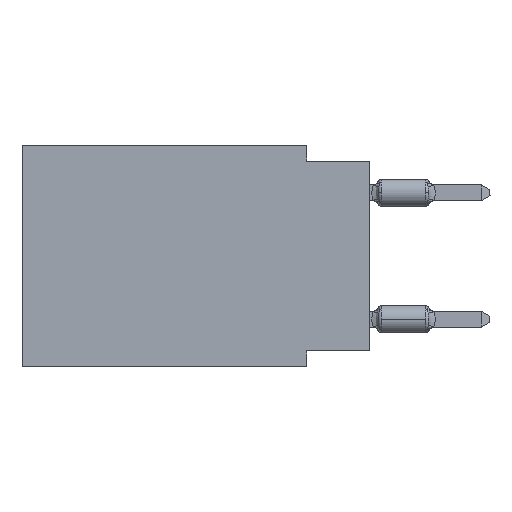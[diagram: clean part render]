
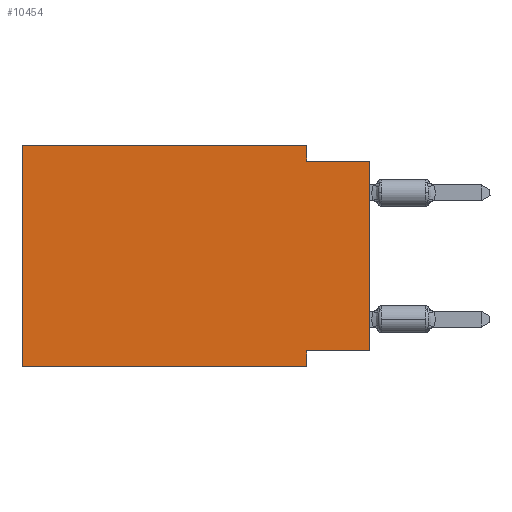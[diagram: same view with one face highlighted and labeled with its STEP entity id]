
A CAD part, left-side view. The second image highlights one B-rep face of the part: STEP entity #10454.
In plain terms, the highlighted planar face has unit normal (-1, 0, 0).
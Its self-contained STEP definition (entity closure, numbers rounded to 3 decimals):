
#143 = VERTEX_POINT ( 'NONE', #18710 ) ;
#406 = LINE ( 'NONE', #12605, #15432 ) ;
#486 = CARTESIAN_POINT ( 'NONE',  ( 0., 0., -0.635 ) ) ;
#492 = VERTEX_POINT ( 'NONE', #29308 ) ;
#1200 = VECTOR ( 'NONE', #30623, 1000. ) ;
#2430 = EDGE_CURVE ( 'NONE', #11170, #37074, #37543, .T. ) ;
#3896 = CARTESIAN_POINT ( 'NONE',  ( 0., 13.97, -8.89 ) ) ;
#4516 = CARTESIAN_POINT ( 'NONE',  ( 0., 0., -8.255 ) ) ;
#5131 = EDGE_CURVE ( 'NONE', #34781, #492, #18862, .T. ) ;
#5402 = AXIS2_PLACEMENT_3D ( 'NONE', #24489, #18121, #9792 ) ;
#5434 = EDGE_LOOP ( 'NONE', ( #22958, #25576, #11327, #9521, #13506, #20418, #31137, #16012 ) ) ;
#5705 = EDGE_CURVE ( 'NONE', #37074, #34781, #22876, .T. ) ;
#5917 = CARTESIAN_POINT ( 'NONE',  ( 0., 13.97, -8.89 ) ) ;
#6017 = CARTESIAN_POINT ( 'NONE',  ( 0., 2.54, -8.89 ) ) ;
#7049 = VERTEX_POINT ( 'NONE', #6017 ) ;
#7102 = EDGE_CURVE ( 'NONE', #143, #7049, #406, .T. ) ;
#8072 = LINE ( 'NONE', #31055, #16519 ) ;
#9521 = ORIENTED_EDGE ( 'NONE', *, *, #2430, .F. ) ;
#9792 = DIRECTION ( 'NONE',  ( 0., 0., -1. ) ) ;
#10207 = CARTESIAN_POINT ( 'NONE',  ( 0., 0., 0. ) ) ;
#10303 = VERTEX_POINT ( 'NONE', #5917 ) ;
#10408 = VECTOR ( 'NONE', #34640, 1000. ) ;
#10454 = ADVANCED_FACE ( 'NONE', ( #32782 ), #12705, .F. ) ;
#10768 = VECTOR ( 'NONE', #13719, 1000. ) ;
#11170 = VERTEX_POINT ( 'NONE', #36300 ) ;
#11327 = ORIENTED_EDGE ( 'NONE', *, *, #5705, .F. ) ;
#12092 = VECTOR ( 'NONE', #13830, 1000. ) ;
#12288 = EDGE_CURVE ( 'NONE', #10303, #7049, #24603, .T. ) ;
#12605 = CARTESIAN_POINT ( 'NONE',  ( 0., 2.54, -8.89 ) ) ;
#12705 = PLANE ( 'NONE',  #5402 ) ;
#13506 = ORIENTED_EDGE ( 'NONE', *, *, #32678, .F. ) ;
#13719 = DIRECTION ( 'NONE',  ( 0., 0., 1. ) ) ;
#13830 = DIRECTION ( 'NONE',  ( 0., 1., 0. ) ) ;
#15386 = CARTESIAN_POINT ( 'NONE',  ( 0., 2.54, 0. ) ) ;
#15432 = VECTOR ( 'NONE', #29792, 1000. ) ;
#16012 = ORIENTED_EDGE ( 'NONE', *, *, #35988, .F. ) ;
#16519 = VECTOR ( 'NONE', #19879, 1000. ) ;
#17059 = CARTESIAN_POINT ( 'NONE',  ( 0., 2.54, 0. ) ) ;
#17237 = VECTOR ( 'NONE', #27504, 1000. ) ;
#18121 = DIRECTION ( 'NONE',  ( 1., 0., 0. ) ) ;
#18710 = CARTESIAN_POINT ( 'NONE',  ( 0., 2.54, -8.255 ) ) ;
#18862 = LINE ( 'NONE', #486, #1200 ) ;
#18929 = VECTOR ( 'NONE', #29420, 1000. ) ;
#19518 = CARTESIAN_POINT ( 'NONE',  ( 0., 0., -8.255 ) ) ;
#19879 = DIRECTION ( 'NONE',  ( 0., 0., 1. ) ) ;
#19963 = VERTEX_POINT ( 'NONE', #19518 ) ;
#20418 = ORIENTED_EDGE ( 'NONE', *, *, #12288, .T. ) ;
#22876 = LINE ( 'NONE', #17059, #10408 ) ;
#22958 = ORIENTED_EDGE ( 'NONE', *, *, #30238, .T. ) ;
#24489 = CARTESIAN_POINT ( 'NONE',  ( 0., 13.97, 0. ) ) ;
#24603 = LINE ( 'NONE', #3896, #17237 ) ;
#25576 = ORIENTED_EDGE ( 'NONE', *, *, #5131, .F. ) ;
#27504 = DIRECTION ( 'NONE',  ( 0., -1., 0. ) ) ;
#29308 = CARTESIAN_POINT ( 'NONE',  ( 0., 0., -0.635 ) ) ;
#29420 = DIRECTION ( 'NONE',  ( 0., -1., 0. ) ) ;
#29792 = DIRECTION ( 'NONE',  ( 0., 0., -1. ) ) ;
#30238 = EDGE_CURVE ( 'NONE', #19963, #492, #31058, .T. ) ;
#30623 = DIRECTION ( 'NONE',  ( 0., -1., 0. ) ) ;
#30785 = CARTESIAN_POINT ( 'NONE',  ( 0., 2.54, -0.635 ) ) ;
#31055 = CARTESIAN_POINT ( 'NONE',  ( 0., 13.97, 0. ) ) ;
#31058 = LINE ( 'NONE', #10207, #10768 ) ;
#31137 = ORIENTED_EDGE ( 'NONE', *, *, #7102, .F. ) ;
#32678 = EDGE_CURVE ( 'NONE', #10303, #11170, #8072, .T. ) ;
#32782 = FACE_OUTER_BOUND ( 'NONE', #5434, .T. ) ;
#34640 = DIRECTION ( 'NONE',  ( 0., 0., -1. ) ) ;
#34781 = VERTEX_POINT ( 'NONE', #30785 ) ;
#34828 = CARTESIAN_POINT ( 'NONE',  ( 0., 13.97, 0. ) ) ;
#35988 = EDGE_CURVE ( 'NONE', #19963, #143, #37169, .T. ) ;
#36300 = CARTESIAN_POINT ( 'NONE',  ( 0., 13.97, 0. ) ) ;
#37074 = VERTEX_POINT ( 'NONE', #15386 ) ;
#37169 = LINE ( 'NONE', #4516, #12092 ) ;
#37543 = LINE ( 'NONE', #34828, #18929 ) ;
